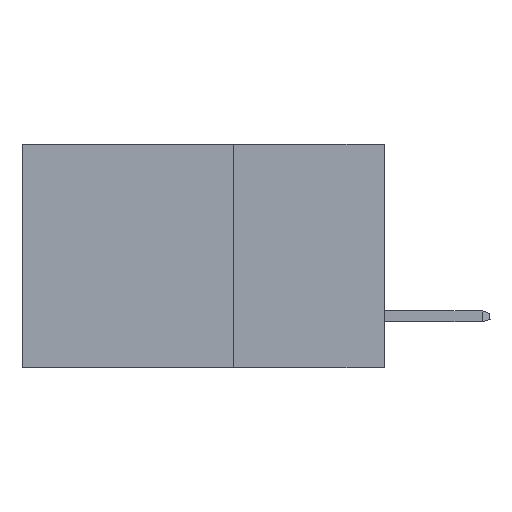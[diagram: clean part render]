
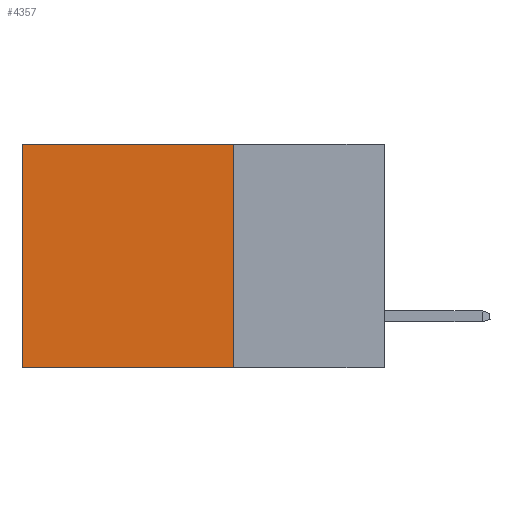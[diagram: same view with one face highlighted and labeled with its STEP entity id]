
A CAD part, left-side view. The second image highlights one B-rep face of the part: STEP entity #4357.
In plain terms, the highlighted planar face has unit normal (-1, 0, 0).
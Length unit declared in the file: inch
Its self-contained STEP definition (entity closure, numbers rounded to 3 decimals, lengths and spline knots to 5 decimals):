
#188 = LINE ( 'NONE', #6371, #2924 ) ;
#732 = CARTESIAN_POINT ( 'NONE',  ( 0.298, 0.25, 0. ) ) ;
#1098 = CARTESIAN_POINT ( 'NONE',  ( 0.298, 0.25, 0. ) ) ;
#1165 = CARTESIAN_POINT ( 'NONE',  ( 0.298, 0.6, 0. ) ) ;
#1287 = VECTOR ( 'NONE', #16953, 39.37008 ) ;
#1385 = LINE ( 'NONE', #13568, #7620 ) ;
#2656 = CARTESIAN_POINT ( 'NONE',  ( 0.298, 0.6, 0. ) ) ;
#2924 = VECTOR ( 'NONE', #17637, 39.37008 ) ;
#3445 = EDGE_CURVE ( 'NONE', #5353, #9290, #188, .T. ) ;
#3847 = VERTEX_POINT ( 'NONE', #15760 ) ;
#4357 = ADVANCED_FACE ( 'NONE', ( #11709 ), #4378, .F. ) ;
#4378 = PLANE ( 'NONE',  #4864 ) ;
#4864 = AXIS2_PLACEMENT_3D ( 'NONE', #1098, #20475, #15466 ) ;
#5353 = VERTEX_POINT ( 'NONE', #732 ) ;
#6036 = LINE ( 'NONE', #11813, #1287 ) ;
#6240 = EDGE_CURVE ( 'NONE', #3847, #12301, #1385, .T. ) ;
#6371 = CARTESIAN_POINT ( 'NONE',  ( 0.298, 0.25, 0. ) ) ;
#7211 = CARTESIAN_POINT ( 'NONE',  ( 0.298, 0.6, -0.37 ) ) ;
#7620 = VECTOR ( 'NONE', #15329, 39.37008 ) ;
#9290 = VERTEX_POINT ( 'NONE', #2656 ) ;
#9797 = EDGE_CURVE ( 'NONE', #9290, #12301, #11420, .T. ) ;
#10650 = DIRECTION ( 'NONE',  ( 0., 0., -1. ) ) ;
#11420 = LINE ( 'NONE', #1165, #12671 ) ;
#11709 = FACE_OUTER_BOUND ( 'NONE', #18310, .T. ) ;
#11813 = CARTESIAN_POINT ( 'NONE',  ( 0.298, 0.25, 0. ) ) ;
#12301 = VERTEX_POINT ( 'NONE', #7211 ) ;
#12671 = VECTOR ( 'NONE', #10650, 39.37008 ) ;
#12745 = ORIENTED_EDGE ( 'NONE', *, *, #9797, .T. ) ;
#13568 = CARTESIAN_POINT ( 'NONE',  ( 0.298, 0.25, -0.37 ) ) ;
#15163 = ORIENTED_EDGE ( 'NONE', *, *, #6240, .F. ) ;
#15329 = DIRECTION ( 'NONE',  ( 0., 1., 0. ) ) ;
#15466 = DIRECTION ( 'NONE',  ( 0., 0., -1. ) ) ;
#15706 = EDGE_CURVE ( 'NONE', #5353, #3847, #6036, .T. ) ;
#15760 = CARTESIAN_POINT ( 'NONE',  ( 0.298, 0.25, -0.37 ) ) ;
#16953 = DIRECTION ( 'NONE',  ( 0., 0., -1. ) ) ;
#17403 = ORIENTED_EDGE ( 'NONE', *, *, #15706, .F. ) ;
#17637 = DIRECTION ( 'NONE',  ( 0., 1., 0. ) ) ;
#18195 = ORIENTED_EDGE ( 'NONE', *, *, #3445, .T. ) ;
#18310 = EDGE_LOOP ( 'NONE', ( #12745, #15163, #17403, #18195 ) ) ;
#20475 = DIRECTION ( 'NONE',  ( 1., 0., 0. ) ) ;
